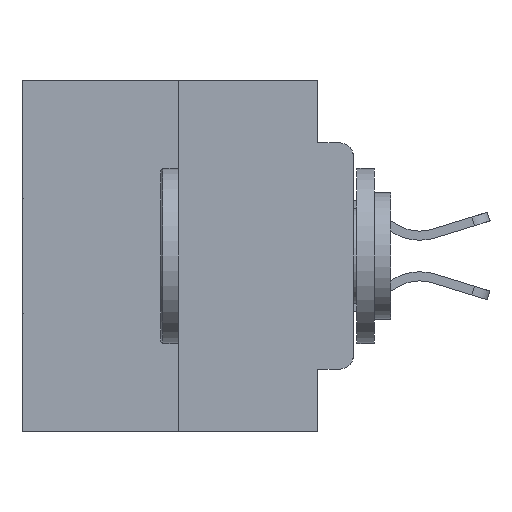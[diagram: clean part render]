
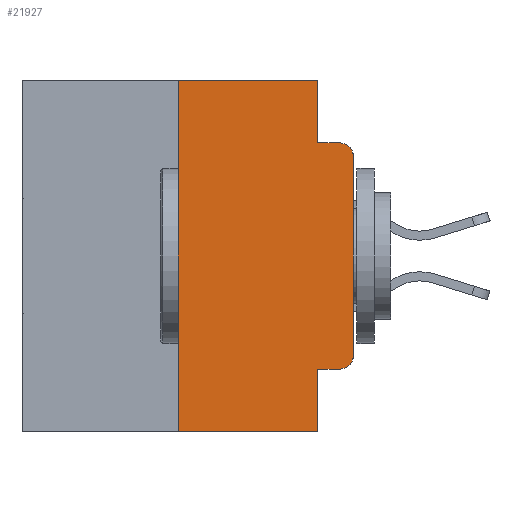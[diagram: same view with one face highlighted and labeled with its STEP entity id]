
A CAD part, left-side view. The second image highlights one B-rep face of the part: STEP entity #21927.
In plain terms, the highlighted planar face has unit normal (-1, 0, 0).
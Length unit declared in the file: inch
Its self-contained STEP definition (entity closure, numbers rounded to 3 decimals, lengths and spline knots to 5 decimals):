
#26 = CARTESIAN_POINT ( 'NONE',  ( 0., 0.25, 0. ) ) ;
#580 = VECTOR ( 'NONE', #1474, 39.37008 ) ;
#940 = DIRECTION ( 'NONE',  ( 0., 0., -1. ) ) ;
#959 = VERTEX_POINT ( 'NONE', #26 ) ;
#1253 = AXIS2_PLACEMENT_3D ( 'NONE', #27652, #14817, #940 ) ;
#1474 = DIRECTION ( 'NONE',  ( 0., 0., 1. ) ) ;
#2360 = CIRCLE ( 'NONE', #24364, 0.02 ) ;
#2889 = VERTEX_POINT ( 'NONE', #19720 ) ;
#3390 = VERTEX_POINT ( 'NONE', #8337 ) ;
#3823 = ORIENTED_EDGE ( 'NONE', *, *, #28017, .T. ) ;
#3889 = ORIENTED_EDGE ( 'NONE', *, *, #23993, .T. ) ;
#4221 = CARTESIAN_POINT ( 'NONE',  ( 0., 0.25, 0. ) ) ;
#4629 = VECTOR ( 'NONE', #10331, 39.37008 ) ;
#5861 = CARTESIAN_POINT ( 'NONE',  ( 0., 0.051, 0. ) ) ;
#6303 = CARTESIAN_POINT ( 'NONE',  ( 0., 0.02, -0.1085 ) ) ;
#7516 = FACE_OUTER_BOUND ( 'NONE', #16297, .T. ) ;
#7797 = CARTESIAN_POINT ( 'NONE',  ( 0., 0.02, -0.4115 ) ) ;
#8337 = CARTESIAN_POINT ( 'NONE',  ( 0., 0.051, -0.5 ) ) ;
#8445 = CARTESIAN_POINT ( 'NONE',  ( 0., 0.051, 0. ) ) ;
#8649 = DIRECTION ( 'NONE',  ( 0., 0., -1. ) ) ;
#9382 = VERTEX_POINT ( 'NONE', #7797 ) ;
#9417 = PLANE ( 'NONE',  #20985 ) ;
#9597 = EDGE_CURVE ( 'NONE', #27436, #24639, #26510, .T. ) ;
#9611 = ORIENTED_EDGE ( 'NONE', *, *, #28776, .F. ) ;
#9691 = ORIENTED_EDGE ( 'NONE', *, *, #22831, .F. ) ;
#9740 = VERTEX_POINT ( 'NONE', #24348 ) ;
#9877 = ORIENTED_EDGE ( 'NONE', *, *, #9597, .T. ) ;
#10223 = CARTESIAN_POINT ( 'NONE',  ( 0., 0.473, 0. ) ) ;
#10243 = CIRCLE ( 'NONE', #1253, 0.02 ) ;
#10331 = DIRECTION ( 'NONE',  ( 0., 0., -1. ) ) ;
#10790 = EDGE_CURVE ( 'NONE', #24724, #9740, #28424, .T. ) ;
#10875 = LINE ( 'NONE', #12402, #16829 ) ;
#11381 = VECTOR ( 'NONE', #12493, 39.37008 ) ;
#11705 = DIRECTION ( 'NONE',  ( 1., 0., 0. ) ) ;
#11780 = ORIENTED_EDGE ( 'NONE', *, *, #10790, .F. ) ;
#12402 = CARTESIAN_POINT ( 'NONE',  ( 0., 0.051, -0.0885 ) ) ;
#12493 = DIRECTION ( 'NONE',  ( 0., -1., 0. ) ) ;
#12697 = CARTESIAN_POINT ( 'NONE',  ( 0., 0., -0.1085 ) ) ;
#13926 = ORIENTED_EDGE ( 'NONE', *, *, #22572, .T. ) ;
#14252 = CARTESIAN_POINT ( 'NONE',  ( 0., 0.25, -0.5 ) ) ;
#14817 = DIRECTION ( 'NONE',  ( -1., 0., 0. ) ) ;
#16031 = DIRECTION ( 'NONE',  ( 0., -1., 0. ) ) ;
#16297 = EDGE_LOOP ( 'NONE', ( #9877, #25620, #9611, #11780, #9691, #24713, #3823, #25054, #13926, #3889 ) ) ;
#16476 = DIRECTION ( 'NONE',  ( 0., -1., 0. ) ) ;
#16789 = EDGE_CURVE ( 'NONE', #26290, #959, #18609, .T. ) ;
#16829 = VECTOR ( 'NONE', #25410, 39.37008 ) ;
#18583 = CARTESIAN_POINT ( 'NONE',  ( 0., 0.473, -0.5 ) ) ;
#18609 = LINE ( 'NONE', #4221, #27937 ) ;
#19053 = VERTEX_POINT ( 'NONE', #25913 ) ;
#19326 = DIRECTION ( 'NONE',  ( 0., 0., -1. ) ) ;
#19696 = EDGE_CURVE ( 'NONE', #2889, #3390, #26104, .T. ) ;
#19720 = CARTESIAN_POINT ( 'NONE',  ( 0., 0.051, -0.4115 ) ) ;
#19992 = DIRECTION ( 'NONE',  ( 0., 0., 1. ) ) ;
#20985 = AXIS2_PLACEMENT_3D ( 'NONE', #24746, #11705, #26877 ) ;
#21684 = EDGE_CURVE ( 'NONE', #24639, #19053, #2360, .T. ) ;
#21905 = DIRECTION ( 'NONE',  ( -1., 0., 0. ) ) ;
#21927 = ADVANCED_FACE ( 'NONE', ( #7516 ), #9417, .F. ) ;
#22572 = EDGE_CURVE ( 'NONE', #2889, #9382, #24696, .T. ) ;
#22800 = VECTOR ( 'NONE', #19326, 39.37008 ) ;
#22831 = EDGE_CURVE ( 'NONE', #959, #24724, #23037, .T. ) ;
#23037 = LINE ( 'NONE', #10223, #11381 ) ;
#23226 = VECTOR ( 'NONE', #16476, 39.37008 ) ;
#23481 = CARTESIAN_POINT ( 'NONE',  ( 0., 0.051, 0. ) ) ;
#23993 = EDGE_CURVE ( 'NONE', #9382, #27436, #10243, .T. ) ;
#24348 = CARTESIAN_POINT ( 'NONE',  ( 0., 0.051, -0.0885 ) ) ;
#24364 = AXIS2_PLACEMENT_3D ( 'NONE', #6303, #21905, #8649 ) ;
#24639 = VERTEX_POINT ( 'NONE', #12697 ) ;
#24696 = LINE ( 'NONE', #28844, #25359 ) ;
#24713 = ORIENTED_EDGE ( 'NONE', *, *, #16789, .F. ) ;
#24724 = VERTEX_POINT ( 'NONE', #8445 ) ;
#24746 = CARTESIAN_POINT ( 'NONE',  ( 0., 0.473, 0. ) ) ;
#24855 = CARTESIAN_POINT ( 'NONE',  ( 0., 0., -0.3915 ) ) ;
#25054 = ORIENTED_EDGE ( 'NONE', *, *, #19696, .F. ) ;
#25359 = VECTOR ( 'NONE', #16031, 39.37008 ) ;
#25410 = DIRECTION ( 'NONE',  ( 0., -1., 0. ) ) ;
#25620 = ORIENTED_EDGE ( 'NONE', *, *, #21684, .T. ) ;
#25913 = CARTESIAN_POINT ( 'NONE',  ( 0., 0.02, -0.0885 ) ) ;
#26104 = LINE ( 'NONE', #23481, #4629 ) ;
#26290 = VERTEX_POINT ( 'NONE', #14252 ) ;
#26510 = LINE ( 'NONE', #28128, #580 ) ;
#26877 = DIRECTION ( 'NONE',  ( 0., 0., -1. ) ) ;
#27436 = VERTEX_POINT ( 'NONE', #24855 ) ;
#27652 = CARTESIAN_POINT ( 'NONE',  ( 0., 0.02, -0.3915 ) ) ;
#27937 = VECTOR ( 'NONE', #19992, 39.37008 ) ;
#28017 = EDGE_CURVE ( 'NONE', #26290, #3390, #28854, .T. ) ;
#28128 = CARTESIAN_POINT ( 'NONE',  ( 0., 0., 0. ) ) ;
#28424 = LINE ( 'NONE', #5861, #22800 ) ;
#28776 = EDGE_CURVE ( 'NONE', #9740, #19053, #10875, .T. ) ;
#28844 = CARTESIAN_POINT ( 'NONE',  ( 0., 0.051, -0.4115 ) ) ;
#28854 = LINE ( 'NONE', #18583, #23226 ) ;
